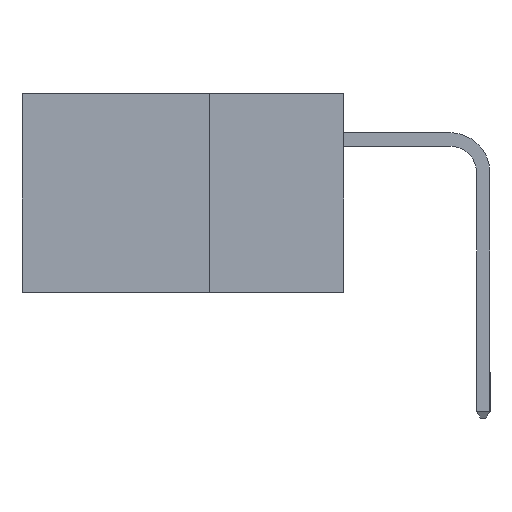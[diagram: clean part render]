
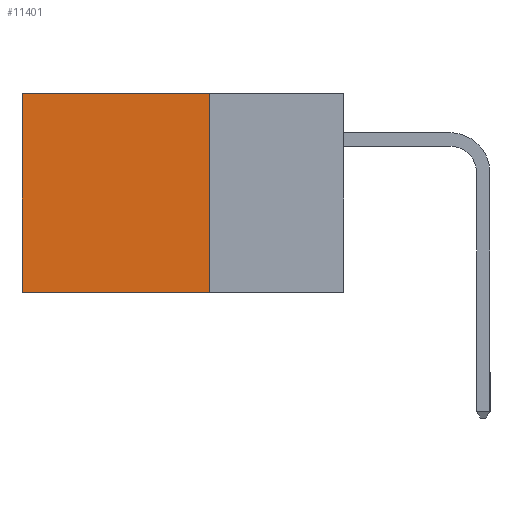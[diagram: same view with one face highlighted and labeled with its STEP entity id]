
A CAD part, left-side view. The second image highlights one B-rep face of the part: STEP entity #11401.
In plain terms, the highlighted planar face has unit normal (-1, 0, 0).
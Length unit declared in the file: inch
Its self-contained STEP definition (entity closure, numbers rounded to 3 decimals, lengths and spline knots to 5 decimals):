
#581 = LINE ( 'NONE', #13052, #3589 ) ;
#694 = DIRECTION ( 'NONE',  ( 0., 0., -1. ) ) ;
#889 = DIRECTION ( 'NONE',  ( 0., 0., -1. ) ) ;
#1550 = ORIENTED_EDGE ( 'NONE', *, *, #13372, .T. ) ;
#1565 = CARTESIAN_POINT ( 'NONE',  ( 0.2615, 0.25, -0.37 ) ) ;
#1741 = AXIS2_PLACEMENT_3D ( 'NONE', #11366, #6920, #8168 ) ;
#1946 = VECTOR ( 'NONE', #694, 39.37008 ) ;
#2129 = CARTESIAN_POINT ( 'NONE',  ( 0.2615, 0.6, 0. ) ) ;
#2503 = PLANE ( 'NONE',  #1741 ) ;
#2663 = LINE ( 'NONE', #12717, #13871 ) ;
#2929 = VERTEX_POINT ( 'NONE', #14366 ) ;
#3516 = ORIENTED_EDGE ( 'NONE', *, *, #10408, .T. ) ;
#3589 = VECTOR ( 'NONE', #9470, 39.37008 ) ;
#3745 = FACE_OUTER_BOUND ( 'NONE', #12142, .T. ) ;
#3828 = CARTESIAN_POINT ( 'NONE',  ( 0.2615, 0.6, -0.37 ) ) ;
#4072 = EDGE_CURVE ( 'NONE', #11278, #9753, #7070, .T. ) ;
#6473 = EDGE_CURVE ( 'NONE', #2929, #11278, #10670, .T. ) ;
#6920 = DIRECTION ( 'NONE',  ( 1., 0., 0. ) ) ;
#7044 = ORIENTED_EDGE ( 'NONE', *, *, #4072, .F. ) ;
#7070 = LINE ( 'NONE', #1565, #13809 ) ;
#7720 = CARTESIAN_POINT ( 'NONE',  ( 0.2615, 0.25, -0.37 ) ) ;
#8168 = DIRECTION ( 'NONE',  ( 0., 0., -1. ) ) ;
#9107 = ORIENTED_EDGE ( 'NONE', *, *, #6473, .F. ) ;
#9470 = DIRECTION ( 'NONE',  ( 0., 1., 0. ) ) ;
#9753 = VERTEX_POINT ( 'NONE', #3828 ) ;
#10408 = EDGE_CURVE ( 'NONE', #2929, #13611, #581, .T. ) ;
#10422 = DIRECTION ( 'NONE',  ( 0., 1., 0. ) ) ;
#10670 = LINE ( 'NONE', #11913, #1946 ) ;
#11278 = VERTEX_POINT ( 'NONE', #7720 ) ;
#11366 = CARTESIAN_POINT ( 'NONE',  ( 0.2615, 0.25, -0.37 ) ) ;
#11401 = ADVANCED_FACE ( 'NONE', ( #3745 ), #2503, .F. ) ;
#11913 = CARTESIAN_POINT ( 'NONE',  ( 0.2615, 0.25, -0.37 ) ) ;
#12142 = EDGE_LOOP ( 'NONE', ( #1550, #7044, #9107, #3516 ) ) ;
#12717 = CARTESIAN_POINT ( 'NONE',  ( 0.2615, 0.6, -0.37 ) ) ;
#13052 = CARTESIAN_POINT ( 'NONE',  ( 0.2615, 0.25, 0. ) ) ;
#13372 = EDGE_CURVE ( 'NONE', #13611, #9753, #2663, .T. ) ;
#13611 = VERTEX_POINT ( 'NONE', #2129 ) ;
#13809 = VECTOR ( 'NONE', #10422, 39.37008 ) ;
#13871 = VECTOR ( 'NONE', #889, 39.37008 ) ;
#14366 = CARTESIAN_POINT ( 'NONE',  ( 0.2615, 0.25, 0. ) ) ;
